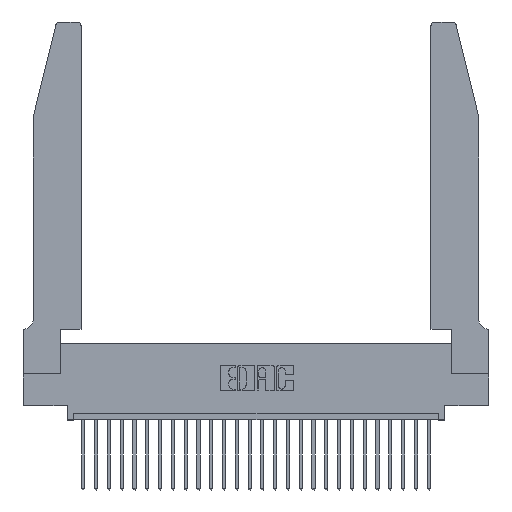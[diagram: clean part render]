
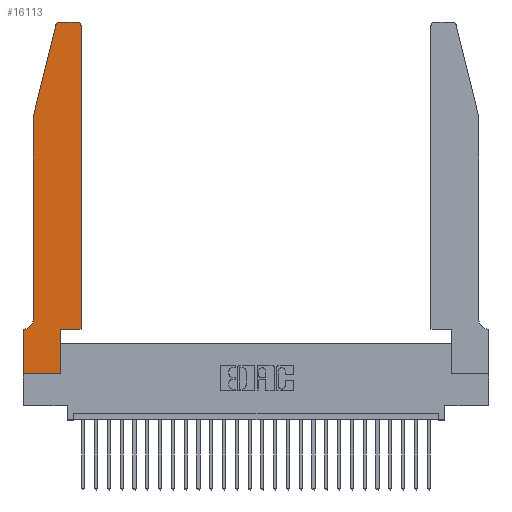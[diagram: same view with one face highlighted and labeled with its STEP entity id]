
A CAD part, top view. The second image highlights one B-rep face of the part: STEP entity #16113.
In plain terms, the highlighted planar face has unit normal (0, 0, 1).
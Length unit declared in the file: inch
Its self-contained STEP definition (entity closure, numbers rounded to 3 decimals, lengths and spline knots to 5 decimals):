
#82 = LINE ( 'NONE', #5575, #15230 ) ;
#259 = LINE ( 'NONE', #14757, #11064 ) ;
#445 = VERTEX_POINT ( 'NONE', #18065 ) ;
#510 = CARTESIAN_POINT ( 'NONE',  ( 0., 0.35, 0.37 ) ) ;
#764 = LINE ( 'NONE', #24509, #10265 ) ;
#1045 = CARTESIAN_POINT ( 'NONE',  ( 0.4505, 0.35, 0.37 ) ) ;
#1586 = ORIENTED_EDGE ( 'NONE', *, *, #15947, .T. ) ;
#1764 = ORIENTED_EDGE ( 'NONE', *, *, #12867, .T. ) ;
#2103 = CARTESIAN_POINT ( 'NONE',  ( 0.0755, 2., 0.37 ) ) ;
#2396 = PLANE ( 'NONE',  #4871 ) ;
#2811 = CARTESIAN_POINT ( 'NONE',  ( 0.4505, 0.35, 0.37 ) ) ;
#3026 = DIRECTION ( 'NONE',  ( 1., 0., 0. ) ) ;
#3070 = VECTOR ( 'NONE', #20327, 39.37008 ) ;
#3910 = LINE ( 'NONE', #3970, #12030 ) ;
#3970 = CARTESIAN_POINT ( 'NONE',  ( 0.0755, 0.35, 0.37 ) ) ;
#4057 = ORIENTED_EDGE ( 'NONE', *, *, #12660, .T. ) ;
#4155 = VECTOR ( 'NONE', #21148, 39.37008 ) ;
#4271 = CARTESIAN_POINT ( 'NONE',  ( 0., 0.35, 0.37 ) ) ;
#4426 = AXIS2_PLACEMENT_3D ( 'NONE', #22229, #22592, #3026 ) ;
#4871 = AXIS2_PLACEMENT_3D ( 'NONE', #4271, #21325, #19332 ) ;
#5130 = CARTESIAN_POINT ( 'NONE',  ( 0.4205, 2.72, 0.37 ) ) ;
#5575 = CARTESIAN_POINT ( 'NONE',  ( 0., 0., 0.37 ) ) ;
#6023 = DIRECTION ( 'NONE',  ( 0., 0., -1. ) ) ;
#6671 = CIRCLE ( 'NONE', #16175, 0.03 ) ;
#8480 = DIRECTION ( 'NONE',  ( -1., 0., 0. ) ) ;
#8754 = CIRCLE ( 'NONE', #4426, 0.03 ) ;
#9583 = EDGE_CURVE ( 'NONE', #18916, #25496, #14815, .T. ) ;
#10038 = ORIENTED_EDGE ( 'NONE', *, *, #12749, .T. ) ;
#10183 = EDGE_LOOP ( 'NONE', ( #11808, #14593, #10038, #19828, #20062, #19838, #4057, #12570, #1764, #18168, #1586, #10206 ) ) ;
#10206 = ORIENTED_EDGE ( 'NONE', *, *, #22681, .T. ) ;
#10265 = VECTOR ( 'NONE', #15694, 39.37008 ) ;
#10462 = VECTOR ( 'NONE', #25546, 39.37008 ) ;
#10463 = VERTEX_POINT ( 'NONE', #12067 ) ;
#10626 = CARTESIAN_POINT ( 'NONE',  ( 0., 0., 0.37 ) ) ;
#10717 = EDGE_CURVE ( 'NONE', #10463, #20970, #3910, .T. ) ;
#10981 = DIRECTION ( 'NONE',  ( 0., 1., 0. ) ) ;
#11006 = CARTESIAN_POINT ( 'NONE',  ( 0.25487, 2.72718, 0.37 ) ) ;
#11064 = VECTOR ( 'NONE', #21252, 39.37008 ) ;
#11448 = VECTOR ( 'NONE', #17488, 39.37008 ) ;
#11537 = VERTEX_POINT ( 'NONE', #26723 ) ;
#11787 = VERTEX_POINT ( 'NONE', #16067 ) ;
#11808 = ORIENTED_EDGE ( 'NONE', *, *, #26096, .T. ) ;
#11979 = DIRECTION ( 'NONE',  ( 1., 0., 0. ) ) ;
#12030 = VECTOR ( 'NONE', #14637, 39.37008 ) ;
#12067 = CARTESIAN_POINT ( 'NONE',  ( 0.0055, 0.35, 0.37 ) ) ;
#12570 = ORIENTED_EDGE ( 'NONE', *, *, #13597, .T. ) ;
#12660 = EDGE_CURVE ( 'NONE', #20970, #17680, #26709, .T. ) ;
#12749 = EDGE_CURVE ( 'NONE', #15631, #445, #764, .T. ) ;
#12867 = EDGE_CURVE ( 'NONE', #25782, #18916, #26054, .T. ) ;
#13159 = VERTEX_POINT ( 'NONE', #22218 ) ;
#13597 = EDGE_CURVE ( 'NONE', #17680, #25782, #82, .T. ) ;
#13694 = CARTESIAN_POINT ( 'NONE',  ( 0.2865, 0.35, 0.37 ) ) ;
#13946 = CIRCLE ( 'NONE', #21860, 0.07 ) ;
#14183 = DIRECTION ( 'NONE',  ( 1., 0., 0. ) ) ;
#14279 = VECTOR ( 'NONE', #10981, 39.37008 ) ;
#14593 = ORIENTED_EDGE ( 'NONE', *, *, #20767, .T. ) ;
#14637 = DIRECTION ( 'NONE',  ( -1., 0., 0. ) ) ;
#14757 = CARTESIAN_POINT ( 'NONE',  ( 0.4505, 0.35, 0.37 ) ) ;
#14815 = LINE ( 'NONE', #2811, #11448 ) ;
#15230 = VECTOR ( 'NONE', #11979, 39.37008 ) ;
#15279 = CARTESIAN_POINT ( 'NONE',  ( 0.2865, 0., 0.37 ) ) ;
#15354 = EDGE_CURVE ( 'NONE', #445, #21596, #15483, .T. ) ;
#15483 = LINE ( 'NONE', #2103, #10462 ) ;
#15631 = VERTEX_POINT ( 'NONE', #11006 ) ;
#15694 = DIRECTION ( 'NONE',  ( -0.239, -0.971, 0. ) ) ;
#15947 = EDGE_CURVE ( 'NONE', #25496, #11787, #259, .T. ) ;
#16067 = CARTESIAN_POINT ( 'NONE',  ( 0.4505, 2.72, 0.37 ) ) ;
#16113 = ADVANCED_FACE ( 'NONE', ( #23519 ), #2396, .T. ) ;
#16175 = AXIS2_PLACEMENT_3D ( 'NONE', #5130, #20286, #14183 ) ;
#17488 = DIRECTION ( 'NONE',  ( 1., 0., 0. ) ) ;
#17680 = VERTEX_POINT ( 'NONE', #10626 ) ;
#17877 = CARTESIAN_POINT ( 'NONE',  ( 0.0755, 0.42, 0.37 ) ) ;
#18023 = EDGE_CURVE ( 'NONE', #21596, #10463, #13946, .T. ) ;
#18065 = CARTESIAN_POINT ( 'NONE',  ( 0.0755, 2., 0.37 ) ) ;
#18168 = ORIENTED_EDGE ( 'NONE', *, *, #9583, .T. ) ;
#18405 = CARTESIAN_POINT ( 'NONE',  ( 0.2605, 2.75, 0.37 ) ) ;
#18916 = VERTEX_POINT ( 'NONE', #13694 ) ;
#19332 = DIRECTION ( 'NONE',  ( 1., 0., 0. ) ) ;
#19828 = ORIENTED_EDGE ( 'NONE', *, *, #15354, .T. ) ;
#19838 = ORIENTED_EDGE ( 'NONE', *, *, #10717, .T. ) ;
#20062 = ORIENTED_EDGE ( 'NONE', *, *, #18023, .T. ) ;
#20286 = DIRECTION ( 'NONE',  ( 0., 0., 1. ) ) ;
#20327 = DIRECTION ( 'NONE',  ( -1., 0., 0. ) ) ;
#20767 = EDGE_CURVE ( 'NONE', #11537, #15631, #8754, .T. ) ;
#20970 = VERTEX_POINT ( 'NONE', #510 ) ;
#21148 = DIRECTION ( 'NONE',  ( 0., -1., 0. ) ) ;
#21252 = DIRECTION ( 'NONE',  ( 0., 1., 0. ) ) ;
#21325 = DIRECTION ( 'NONE',  ( 0., 0., 1. ) ) ;
#21596 = VERTEX_POINT ( 'NONE', #17877 ) ;
#21860 = AXIS2_PLACEMENT_3D ( 'NONE', #27850, #6023, #8480 ) ;
#22218 = CARTESIAN_POINT ( 'NONE',  ( 0.4205, 2.75, 0.37 ) ) ;
#22229 = CARTESIAN_POINT ( 'NONE',  ( 0.284, 2.72, 0.37 ) ) ;
#22592 = DIRECTION ( 'NONE',  ( 0., 0., 1. ) ) ;
#22681 = EDGE_CURVE ( 'NONE', #11787, #13159, #6671, .T. ) ;
#23519 = FACE_OUTER_BOUND ( 'NONE', #10183, .T. ) ;
#23748 = CARTESIAN_POINT ( 'NONE',  ( 0.2865, 0.35, 0.37 ) ) ;
#24509 = CARTESIAN_POINT ( 'NONE',  ( 0.0755, 2., 0.37 ) ) ;
#25496 = VERTEX_POINT ( 'NONE', #1045 ) ;
#25546 = DIRECTION ( 'NONE',  ( 0., -1., 0. ) ) ;
#25578 = CARTESIAN_POINT ( 'NONE',  ( 0., 0., 0.37 ) ) ;
#25782 = VERTEX_POINT ( 'NONE', #15279 ) ;
#26054 = LINE ( 'NONE', #23748, #14279 ) ;
#26096 = EDGE_CURVE ( 'NONE', #13159, #11537, #26328, .T. ) ;
#26328 = LINE ( 'NONE', #18405, #3070 ) ;
#26709 = LINE ( 'NONE', #25578, #4155 ) ;
#26723 = CARTESIAN_POINT ( 'NONE',  ( 0.284, 2.75, 0.37 ) ) ;
#27850 = CARTESIAN_POINT ( 'NONE',  ( 0.0055, 0.42, 0.37 ) ) ;
